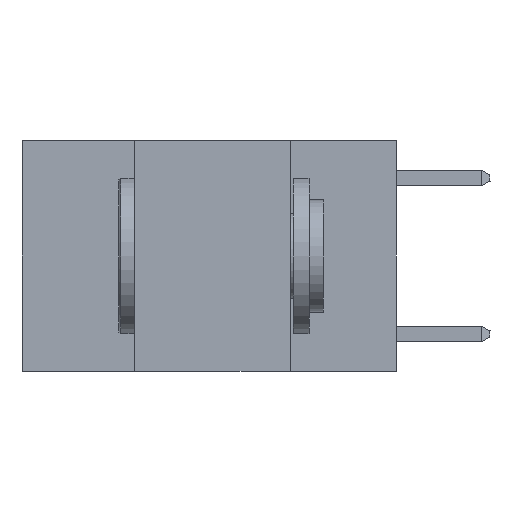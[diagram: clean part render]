
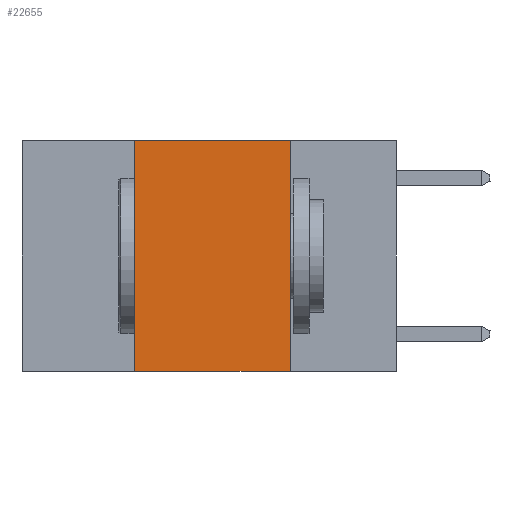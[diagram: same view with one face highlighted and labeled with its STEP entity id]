
A CAD part, left-side view. The second image highlights one B-rep face of the part: STEP entity #22655.
In plain terms, the highlighted planar face has unit normal (-1, 0, 0).
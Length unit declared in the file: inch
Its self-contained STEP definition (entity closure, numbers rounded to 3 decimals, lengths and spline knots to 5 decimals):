
#680 = EDGE_CURVE ( 'NONE', #18660, #27646, #19855, .T. ) ;
#820 = VERTEX_POINT ( 'NONE', #2943 ) ;
#1326 = CARTESIAN_POINT ( 'NONE',  ( 0., 0.42, -0.37 ) ) ;
#1515 = LINE ( 'NONE', #22267, #10273 ) ;
#1656 = DIRECTION ( 'NONE',  ( 0., 0., -1. ) ) ;
#1703 = VECTOR ( 'NONE', #13199, 39.37008 ) ;
#2051 = EDGE_CURVE ( 'NONE', #27646, #820, #29642, .T. ) ;
#2407 = CARTESIAN_POINT ( 'NONE',  ( 0., 0.17, -0.37 ) ) ;
#2943 = CARTESIAN_POINT ( 'NONE',  ( 0., 0.17, 0. ) ) ;
#4759 = PLANE ( 'NONE',  #17189 ) ;
#6564 = LINE ( 'NONE', #20263, #1703 ) ;
#7453 = CARTESIAN_POINT ( 'NONE',  ( 0., 0.6, 0. ) ) ;
#8417 = CARTESIAN_POINT ( 'NONE',  ( 0., 0.42, 0. ) ) ;
#10010 = DIRECTION ( 'NONE',  ( 1., 0., 0. ) ) ;
#10109 = EDGE_LOOP ( 'NONE', ( #27417, #16647, #21260, #11509 ) ) ;
#10273 = VECTOR ( 'NONE', #1656, 39.37008 ) ;
#11296 = CARTESIAN_POINT ( 'NONE',  ( 0., 0.6, 0. ) ) ;
#11509 = ORIENTED_EDGE ( 'NONE', *, *, #20057, .T. ) ;
#12281 = FACE_OUTER_BOUND ( 'NONE', #10109, .T. ) ;
#12797 = DIRECTION ( 'NONE',  ( 0., 0., 1. ) ) ;
#13199 = DIRECTION ( 'NONE',  ( 0., -1., 0. ) ) ;
#14679 = VECTOR ( 'NONE', #26626, 39.37008 ) ;
#16325 = EDGE_CURVE ( 'NONE', #820, #23587, #1515, .T. ) ;
#16647 = ORIENTED_EDGE ( 'NONE', *, *, #2051, .F. ) ;
#17133 = VECTOR ( 'NONE', #12797, 39.37008 ) ;
#17189 = AXIS2_PLACEMENT_3D ( 'NONE', #7453, #10010, #21299 ) ;
#18660 = VERTEX_POINT ( 'NONE', #1326 ) ;
#19855 = LINE ( 'NONE', #8417, #17133 ) ;
#20057 = EDGE_CURVE ( 'NONE', #18660, #23587, #6564, .T. ) ;
#20263 = CARTESIAN_POINT ( 'NONE',  ( 0., 0.6, -0.37 ) ) ;
#21260 = ORIENTED_EDGE ( 'NONE', *, *, #680, .F. ) ;
#21299 = DIRECTION ( 'NONE',  ( 0., 0., -1. ) ) ;
#22267 = CARTESIAN_POINT ( 'NONE',  ( 0., 0.17, 0. ) ) ;
#22655 = ADVANCED_FACE ( 'NONE', ( #12281 ), #4759, .F. ) ;
#23587 = VERTEX_POINT ( 'NONE', #2407 ) ;
#25399 = CARTESIAN_POINT ( 'NONE',  ( 0., 0.42, 0. ) ) ;
#26626 = DIRECTION ( 'NONE',  ( 0., -1., 0. ) ) ;
#27417 = ORIENTED_EDGE ( 'NONE', *, *, #16325, .F. ) ;
#27646 = VERTEX_POINT ( 'NONE', #25399 ) ;
#29642 = LINE ( 'NONE', #11296, #14679 ) ;
